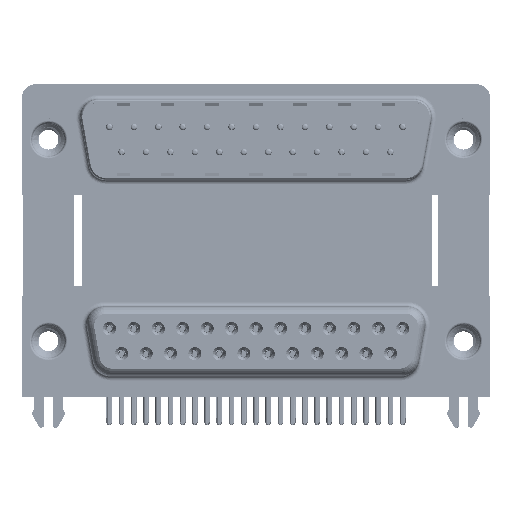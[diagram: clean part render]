
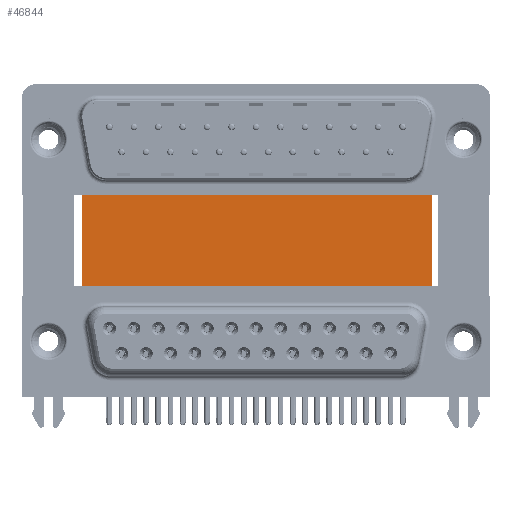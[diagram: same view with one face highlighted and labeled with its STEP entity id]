
A CAD part, top view. The second image highlights one B-rep face of the part: STEP entity #46844.
In plain terms, the highlighted planar face has unit normal (0, 0, 1).
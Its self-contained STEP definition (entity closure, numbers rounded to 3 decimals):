
#175 = DIRECTION ( 'NONE',  ( 0., -1., 0. ) ) ;
#1092 = CARTESIAN_POINT ( 'NONE',  ( 43.43, -3.735, -12. ) ) ;
#2040 = DIRECTION ( 'NONE',  ( -1., 0., 0. ) ) ;
#4492 = LINE ( 'NONE', #39978, #33930 ) ;
#5021 = CARTESIAN_POINT ( 'NONE',  ( 3.79, -3.735, -12. ) ) ;
#5947 = VECTOR ( 'NONE', #27832, 1000. ) ;
#6012 = LINE ( 'NONE', #15021, #5947 ) ;
#8540 = CARTESIAN_POINT ( 'NONE',  ( 3.79, 16.585, -12. ) ) ;
#10570 = CARTESIAN_POINT ( 'NONE',  ( 3.79, 16.585, -12. ) ) ;
#11344 = CARTESIAN_POINT ( 'NONE',  ( 3.79, 16.585, -12. ) ) ;
#11601 = ORIENTED_EDGE ( 'NONE', *, *, #39031, .F. ) ;
#14254 = VERTEX_POINT ( 'NONE', #1092 ) ;
#14722 = EDGE_CURVE ( 'NONE', #18448, #14254, #4492, .T. ) ;
#15021 = CARTESIAN_POINT ( 'NONE',  ( 3.79, 16.585, -12. ) ) ;
#16359 = VERTEX_POINT ( 'NONE', #5021 ) ;
#16932 = VECTOR ( 'NONE', #34700, 1000. ) ;
#18448 = VERTEX_POINT ( 'NONE', #35462 ) ;
#19215 = VERTEX_POINT ( 'NONE', #10570 ) ;
#21326 = VECTOR ( 'NONE', #55091, 1000. ) ;
#22153 = ORIENTED_EDGE ( 'NONE', *, *, #27053, .T. ) ;
#23140 = ORIENTED_EDGE ( 'NONE', *, *, #34023, .T. ) ;
#25274 = DIRECTION ( 'NONE',  ( 0., 0., -1. ) ) ;
#27053 = EDGE_CURVE ( 'NONE', #19215, #16359, #6012, .T. ) ;
#27832 = DIRECTION ( 'NONE',  ( 0., -1., 0. ) ) ;
#31814 = AXIS2_PLACEMENT_3D ( 'NONE', #11344, #25274, #2040 ) ;
#32140 = LINE ( 'NONE', #36505, #21326 ) ;
#33930 = VECTOR ( 'NONE', #175, 1000. ) ;
#34023 = EDGE_CURVE ( 'NONE', #16359, #14254, #32140, .T. ) ;
#34700 = DIRECTION ( 'NONE',  ( 1., 0., 0. ) ) ;
#35462 = CARTESIAN_POINT ( 'NONE',  ( 43.43, 16.585, -12. ) ) ;
#36505 = CARTESIAN_POINT ( 'NONE',  ( 3.79, -3.735, -12. ) ) ;
#39031 = EDGE_CURVE ( 'NONE', #19215, #18448, #43730, .T. ) ;
#39978 = CARTESIAN_POINT ( 'NONE',  ( 43.43, 16.585, -12. ) ) ;
#41877 = FACE_OUTER_BOUND ( 'NONE', #55082, .T. ) ;
#43730 = LINE ( 'NONE', #8540, #16932 ) ;
#46844 = ADVANCED_FACE ( 'NONE', ( #41877 ), #50887, .F. ) ;
#48901 = ORIENTED_EDGE ( 'NONE', *, *, #14722, .F. ) ;
#50887 = PLANE ( 'NONE',  #31814 ) ;
#55082 = EDGE_LOOP ( 'NONE', ( #23140, #48901, #11601, #22153 ) ) ;
#55091 = DIRECTION ( 'NONE',  ( 1., 0., 0. ) ) ;
